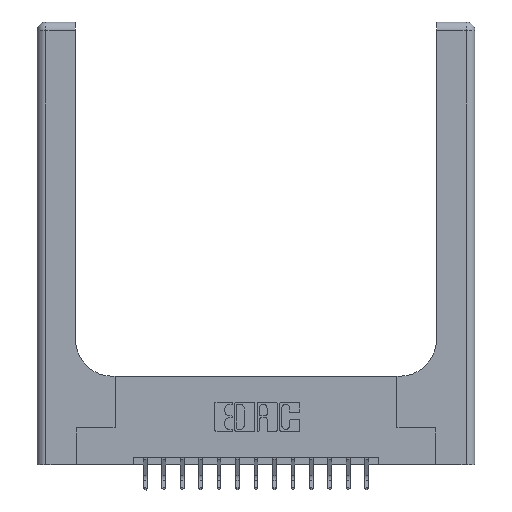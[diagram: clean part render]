
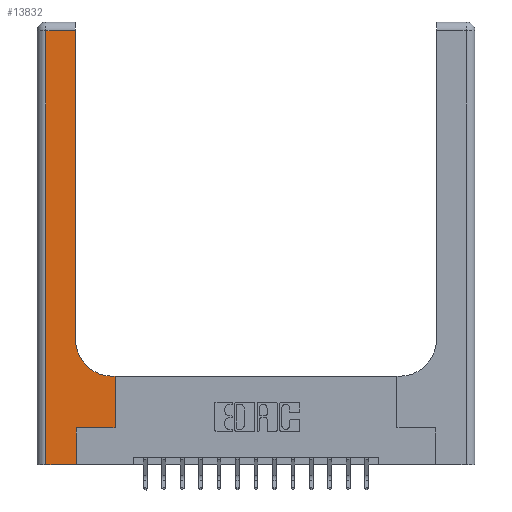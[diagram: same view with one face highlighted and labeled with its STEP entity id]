
A CAD part, top view. The second image highlights one B-rep face of the part: STEP entity #13832.
In plain terms, the highlighted planar face has unit normal (0, 0, 1).
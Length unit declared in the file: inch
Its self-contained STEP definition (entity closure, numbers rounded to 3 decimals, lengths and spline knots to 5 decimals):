
#16 = DIRECTION ( 'NONE',  ( -1., 0., 0. ) ) ;
#432 = VECTOR ( 'NONE', #16, 39.37008 ) ;
#699 = ORIENTED_EDGE ( 'NONE', *, *, #5631, .T. ) ;
#884 = CARTESIAN_POINT ( 'NONE',  ( 0., 0., 0.37 ) ) ;
#940 = CARTESIAN_POINT ( 'NONE',  ( 0.26, 3., 0.37 ) ) ;
#1254 = ORIENTED_EDGE ( 'NONE', *, *, #4172, .T. ) ;
#1255 = CARTESIAN_POINT ( 'NONE',  ( 0.06, 3., 0.37 ) ) ;
#1492 = VERTEX_POINT ( 'NONE', #13802 ) ;
#1626 = VECTOR ( 'NONE', #1751, 39.37008 ) ;
#1751 = DIRECTION ( 'NONE',  ( -1., 0., 0. ) ) ;
#1764 = EDGE_CURVE ( 'NONE', #16292, #3292, #12018, .T. ) ;
#1934 = DIRECTION ( 'NONE',  ( 0., 0., -1. ) ) ;
#2016 = VECTOR ( 'NONE', #2500, 39.37008 ) ;
#2256 = CARTESIAN_POINT ( 'NONE',  ( 0.06, 0., 0.37 ) ) ;
#2329 = EDGE_CURVE ( 'NONE', #1492, #16292, #5127, .T. ) ;
#2500 = DIRECTION ( 'NONE',  ( 0., -1., 0. ) ) ;
#2680 = CARTESIAN_POINT ( 'NONE',  ( 0.26, 0.85, 0.37 ) ) ;
#2920 = LINE ( 'NONE', #884, #13491 ) ;
#3292 = VERTEX_POINT ( 'NONE', #14733 ) ;
#3507 = ORIENTED_EDGE ( 'NONE', *, *, #12929, .T. ) ;
#3668 = ORIENTED_EDGE ( 'NONE', *, *, #15799, .T. ) ;
#4014 = CARTESIAN_POINT ( 'NONE',  ( 0., 3., 0.37 ) ) ;
#4172 = EDGE_CURVE ( 'NONE', #13679, #7180, #10814, .T. ) ;
#4208 = EDGE_LOOP ( 'NONE', ( #15321, #3668, #10716, #699, #10199, #1254, #3507, #6727, #13223 ) ) ;
#4260 = EDGE_CURVE ( 'NONE', #11261, #13679, #6860, .T. ) ;
#4656 = VERTEX_POINT ( 'NONE', #12148 ) ;
#4831 = CARTESIAN_POINT ( 'NONE',  ( 0.265, 0., 0.37 ) ) ;
#5026 = DIRECTION ( 'NONE',  ( 1., 0., 0. ) ) ;
#5127 = CIRCLE ( 'NONE', #8128, 0.25 ) ;
#5287 = VECTOR ( 'NONE', #9471, 39.37008 ) ;
#5399 = CARTESIAN_POINT ( 'NONE',  ( 0.265, 0.25, 0.37 ) ) ;
#5491 = DIRECTION ( 'NONE',  ( 0., 0., -1. ) ) ;
#5631 = EDGE_CURVE ( 'NONE', #8973, #11261, #2920, .T. ) ;
#6249 = EDGE_CURVE ( 'NONE', #4656, #1492, #13683, .T. ) ;
#6724 = CARTESIAN_POINT ( 'NONE',  ( 0.265, 0.25, 0.37 ) ) ;
#6727 = ORIENTED_EDGE ( 'NONE', *, *, #6249, .T. ) ;
#6860 = LINE ( 'NONE', #8475, #9649 ) ;
#7180 = VERTEX_POINT ( 'NONE', #11450 ) ;
#7186 = CARTESIAN_POINT ( 'NONE',  ( 0.06, 2.94, 0.37 ) ) ;
#7477 = LINE ( 'NONE', #16478, #432 ) ;
#7981 = LINE ( 'NONE', #1255, #2016 ) ;
#8014 = VECTOR ( 'NONE', #16553, 39.37008 ) ;
#8128 = AXIS2_PLACEMENT_3D ( 'NONE', #12440, #1934, #15755 ) ;
#8436 = LINE ( 'NONE', #10932, #8014 ) ;
#8475 = CARTESIAN_POINT ( 'NONE',  ( 0.265, 0., 0.37 ) ) ;
#8973 = VERTEX_POINT ( 'NONE', #2256 ) ;
#9471 = DIRECTION ( 'NONE',  ( 0., 1., 0. ) ) ;
#9649 = VECTOR ( 'NONE', #15394, 39.37008 ) ;
#10199 = ORIENTED_EDGE ( 'NONE', *, *, #4260, .T. ) ;
#10716 = ORIENTED_EDGE ( 'NONE', *, *, #13735, .T. ) ;
#10814 = LINE ( 'NONE', #5399, #11248 ) ;
#10932 = CARTESIAN_POINT ( 'NONE',  ( 0.528, 0.25, 0.37 ) ) ;
#11248 = VECTOR ( 'NONE', #13896, 39.37008 ) ;
#11261 = VERTEX_POINT ( 'NONE', #4831 ) ;
#11450 = CARTESIAN_POINT ( 'NONE',  ( 0.528, 0.25, 0.37 ) ) ;
#12018 = LINE ( 'NONE', #940, #5287 ) ;
#12148 = CARTESIAN_POINT ( 'NONE',  ( 0.528, 0.6, 0.37 ) ) ;
#12194 = PLANE ( 'NONE',  #14289 ) ;
#12440 = CARTESIAN_POINT ( 'NONE',  ( 0.51, 0.85, 0.37 ) ) ;
#12743 = CARTESIAN_POINT ( 'NONE',  ( 0.26, 0.6, 0.37 ) ) ;
#12929 = EDGE_CURVE ( 'NONE', #7180, #4656, #8436, .T. ) ;
#13223 = ORIENTED_EDGE ( 'NONE', *, *, #2329, .T. ) ;
#13491 = VECTOR ( 'NONE', #5026, 39.37008 ) ;
#13679 = VERTEX_POINT ( 'NONE', #6724 ) ;
#13683 = LINE ( 'NONE', #12743, #1626 ) ;
#13735 = EDGE_CURVE ( 'NONE', #16448, #8973, #7981, .T. ) ;
#13802 = CARTESIAN_POINT ( 'NONE',  ( 0.51, 0.6, 0.37 ) ) ;
#13832 = ADVANCED_FACE ( 'NONE', ( #14055 ), #12194, .F. ) ;
#13896 = DIRECTION ( 'NONE',  ( 1., 0., 0. ) ) ;
#14055 = FACE_OUTER_BOUND ( 'NONE', #4208, .T. ) ;
#14289 = AXIS2_PLACEMENT_3D ( 'NONE', #4014, #5491, #15164 ) ;
#14733 = CARTESIAN_POINT ( 'NONE',  ( 0.26, 2.94, 0.37 ) ) ;
#15164 = DIRECTION ( 'NONE',  ( -1., 0., 0. ) ) ;
#15321 = ORIENTED_EDGE ( 'NONE', *, *, #1764, .T. ) ;
#15394 = DIRECTION ( 'NONE',  ( 0., 1., 0. ) ) ;
#15755 = DIRECTION ( 'NONE',  ( 1., 0., 0. ) ) ;
#15799 = EDGE_CURVE ( 'NONE', #3292, #16448, #7477, .T. ) ;
#16292 = VERTEX_POINT ( 'NONE', #2680 ) ;
#16448 = VERTEX_POINT ( 'NONE', #7186 ) ;
#16478 = CARTESIAN_POINT ( 'NONE',  ( 0., 2.94, 0.37 ) ) ;
#16553 = DIRECTION ( 'NONE',  ( 0., 1., 0. ) ) ;
